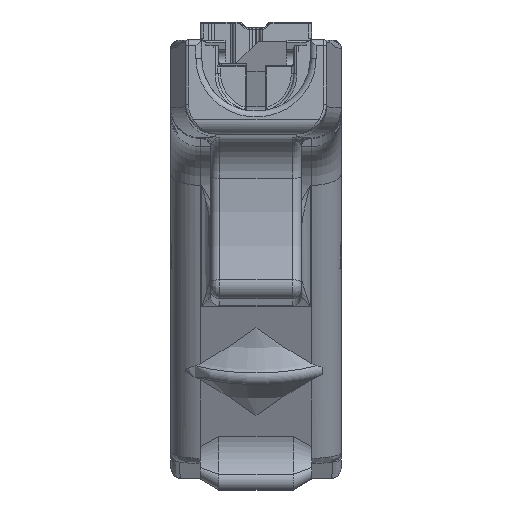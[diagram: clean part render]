
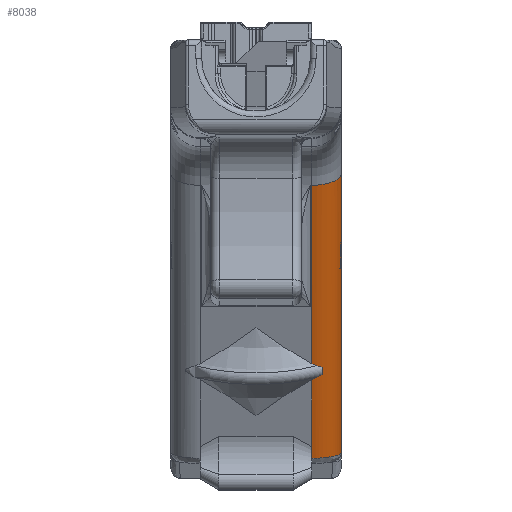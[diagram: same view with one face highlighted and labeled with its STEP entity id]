
A CAD part, top view. The second image highlights one B-rep face of the part: STEP entity #8038.
In plain terms, the highlighted cylindrical face has radius 5.08 mm (diameter 10.16 mm), a partial arc.
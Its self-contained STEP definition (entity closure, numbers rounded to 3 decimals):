
#89=(
BOUNDED_CURVE()
B_SPLINE_CURVE(3,(#33505,#33506,#33507,#33508,#33509,#33510,#33511,#33512,
#33513,#33514),.UNSPECIFIED.,.F.,.F.)
B_SPLINE_CURVE_WITH_KNOTS((4,2,2,2,4),(0.,0.393,0.785,
1.178,1.571),.UNSPECIFIED.)
CURVE()
GEOMETRIC_REPRESENTATION_ITEM()
RATIONAL_B_SPLINE_CURVE((1.,1.,1.,1.,1.,1.,1.,1.,1.,1.))
REPRESENTATION_ITEM('')
);
#125=ELLIPSE('',#8392,5.11,5.08);
#160=ELLIPSE('',#8741,46.774,5.08);
#799=LINE('',#29656,#1373);
#800=LINE('',#29658,#1374);
#846=LINE('',#32326,#1420);
#848=LINE('',#32330,#1422);
#899=LINE('',#33502,#1473);
#900=LINE('',#33504,#1474);
#1373=VECTOR('',#10200,1000.);
#1374=VECTOR('',#10201,1000.);
#1420=VECTOR('',#10403,1000.);
#1422=VECTOR('',#10407,1000.);
#1473=VECTOR('',#10572,1000.);
#1474=VECTOR('',#10573,1000.);
#1621=CYLINDRICAL_SURFACE('',#8740,5.08);
#1986=FACE_OUTER_BOUND('',#2454,.T.);
#2454=EDGE_LOOP('',(#7122,#7123,#7124,#7125,#7126,#7127,#7128,#7129,#7130,
#7131,#7132,#7133,#7134,#7135,#7136));
#2663=CIRCLE('',#8394,5.14);
#2814=CIRCLE('',#8739,5.08);
#3076=B_SPLINE_CURVE_WITH_KNOTS('',3,(#31899,#31900,#31901,#31902),
 .UNSPECIFIED.,.F.,.F.,(4,4),(3.929,4.031),
 .UNSPECIFIED.);
#3077=B_SPLINE_CURVE_WITH_KNOTS('',3,(#31905,#31906,#31907,#31908,#31909,
#31910),.UNSPECIFIED.,.F.,.F.,(4,2,4),(-0.097,-0.066,
-0.064),.UNSPECIFIED.);
#3078=B_SPLINE_CURVE_WITH_KNOTS('',3,(#31914,#31915,#31916,#31917,#31918,
#31919),.UNSPECIFIED.,.F.,.F.,(4,2,4),(-0.485,-0.459,
-0.454),.UNSPECIFIED.);
#3083=B_SPLINE_CURVE_WITH_KNOTS('',3,(#31967,#31968,#31969,#31970,#31971,
#31972),.UNSPECIFIED.,.F.,.F.,(4,2,4),(2.418,2.421,
2.517),.UNSPECIFIED.);
#3503=VERTEX_POINT('',#28126);
#3504=VERTEX_POINT('',#28128);
#3505=VERTEX_POINT('',#28132);
#3506=VERTEX_POINT('',#28134);
#3726=VERTEX_POINT('',#29654);
#3727=VERTEX_POINT('',#29657);
#3800=VERTEX_POINT('',#31878);
#3803=VERTEX_POINT('',#31892);
#3804=VERTEX_POINT('',#31904);
#3805=VERTEX_POINT('',#31911);
#3806=VERTEX_POINT('',#31913);
#3809=VERTEX_POINT('',#31949);
#3818=VERTEX_POINT('',#32324);
#3819=VERTEX_POINT('',#32329);
#3890=VERTEX_POINT('',#33503);
#4439=EDGE_CURVE('',#3503,#3504,#125,.T.);
#4442=EDGE_CURVE('',#3505,#3506,#2663,.T.);
#4789=EDGE_CURVE('',#3726,#3505,#799,.T.);
#4790=EDGE_CURVE('',#3504,#3727,#800,.T.);
#4893=EDGE_CURVE('',#3803,#3800,#3076,.T.);
#4894=EDGE_CURVE('',#3800,#3804,#3077,.T.);
#4896=EDGE_CURVE('',#3805,#3806,#3078,.T.);
#4902=EDGE_CURVE('',#3806,#3809,#3083,.T.);
#4922=EDGE_CURVE('',#3818,#3803,#846,.T.);
#4924=EDGE_CURVE('',#3809,#3819,#848,.T.);
#5033=EDGE_CURVE('',#3726,#3819,#2814,.T.);
#5034=EDGE_CURVE('',#3805,#3804,#899,.T.);
#5035=EDGE_CURVE('',#3890,#3818,#900,.T.);
#5036=EDGE_CURVE('',#3890,#3727,#89,.T.);
#5037=EDGE_CURVE('',#3506,#3503,#160,.T.);
#7122=ORIENTED_EDGE('',*,*,#4442,.F.);
#7123=ORIENTED_EDGE('',*,*,#4789,.F.);
#7124=ORIENTED_EDGE('',*,*,#5033,.T.);
#7125=ORIENTED_EDGE('',*,*,#4924,.F.);
#7126=ORIENTED_EDGE('',*,*,#4902,.F.);
#7127=ORIENTED_EDGE('',*,*,#4896,.F.);
#7128=ORIENTED_EDGE('',*,*,#5034,.T.);
#7129=ORIENTED_EDGE('',*,*,#4894,.F.);
#7130=ORIENTED_EDGE('',*,*,#4893,.F.);
#7131=ORIENTED_EDGE('',*,*,#4922,.F.);
#7132=ORIENTED_EDGE('',*,*,#5035,.F.);
#7133=ORIENTED_EDGE('',*,*,#5036,.T.);
#7134=ORIENTED_EDGE('',*,*,#4790,.F.);
#7135=ORIENTED_EDGE('',*,*,#4439,.F.);
#7136=ORIENTED_EDGE('',*,*,#5037,.F.);
#8038=ADVANCED_FACE('',(#1986),#1621,.T.);
#8392=AXIS2_PLACEMENT_3D('',#28129,#9583,#9584);
#8394=AXIS2_PLACEMENT_3D('',#28135,#9589,#9590);
#8739=AXIS2_PLACEMENT_3D('',#33500,#10568,#10569);
#8740=AXIS2_PLACEMENT_3D('',#33501,#10570,#10571);
#8741=AXIS2_PLACEMENT_3D('',#33515,#10574,#10575);
#9583=DIRECTION('center_axis',(0.,0.952,0.305));
#9584=DIRECTION('ref_axis',(0.,-0.305,0.952));
#9589=DIRECTION('center_axis',(0.,-0.952,
-0.305));
#9590=DIRECTION('ref_axis',(0.995,-0.03,0.093));
#10200=DIRECTION('',(0.,-0.914,-0.407));
#10201=DIRECTION('',(0.,-0.914,-0.407));
#10403=DIRECTION('',(0.,0.914,0.407));
#10407=DIRECTION('',(0.,0.914,0.407));
#10568=DIRECTION('center_axis',(0.,-0.914,-0.407));
#10569=DIRECTION('ref_axis',(0.,0.407,-0.914));
#10570=DIRECTION('center_axis',(0.,0.914,0.407));
#10571=DIRECTION('ref_axis',(0.,-0.407,0.914));
#10572=DIRECTION('',(0.,-0.914,-0.407));
#10573=DIRECTION('',(0.,0.914,0.407));
#10574=DIRECTION('center_axis',(0.,0.305,
-0.952));
#10575=DIRECTION('ref_axis',(0.,0.952,0.305));
#28126=CARTESIAN_POINT('',(14.424,-38.99,-96.538));
#28128=CARTESIAN_POINT('',(14.605,-38.578,-97.825));
#28129=CARTESIAN_POINT('Origin',(9.525,-38.578,-97.825));
#28132=CARTESIAN_POINT('',(14.605,-31.459,-94.656));
#28134=CARTESIAN_POINT('',(14.58,-31.613,-94.175));
#28135=CARTESIAN_POINT('Origin',(9.465,-31.459,-94.656));
#29654=CARTESIAN_POINT('',(14.605,-22.676,-90.746));
#29656=CARTESIAN_POINT('',(14.605,-70.324,-111.956));
#29657=CARTESIAN_POINT('',(14.605,-70.353,-111.969));
#29658=CARTESIAN_POINT('',(14.605,-70.324,-111.956));
#31878=CARTESIAN_POINT('',(10.428,-57.542,-100.794));
#31892=CARTESIAN_POINT('',(9.525,-57.963,-100.893));
#31899=CARTESIAN_POINT('Ctrl Pts',(9.525,-57.963,-100.893));
#31900=CARTESIAN_POINT('Ctrl Pts',(9.817,-57.812,-100.826));
#31901=CARTESIAN_POINT('Ctrl Pts',(10.12,-57.673,-100.792));
#31902=CARTESIAN_POINT('Ctrl Pts',(10.428,-57.542,-100.794));
#31904=CARTESIAN_POINT('',(11.329,-57.063,-100.855));
#31905=CARTESIAN_POINT('Ctrl Pts',(10.428,-57.542,-100.794));
#31906=CARTESIAN_POINT('Ctrl Pts',(10.749,-57.405,-100.797));
#31907=CARTESIAN_POINT('Ctrl Pts',(11.038,-57.249,-100.82));
#31908=CARTESIAN_POINT('Ctrl Pts',(11.298,-57.082,-100.851));
#31909=CARTESIAN_POINT('Ctrl Pts',(11.314,-57.073,-100.853));
#31910=CARTESIAN_POINT('Ctrl Pts',(11.329,-57.063,-100.855));
#31911=CARTESIAN_POINT('',(11.329,-55.855,-100.317));
#31913=CARTESIAN_POINT('',(10.428,-55.58,-99.921));
#31914=CARTESIAN_POINT('Ctrl Pts',(11.329,-55.855,-100.317));
#31915=CARTESIAN_POINT('Ctrl Pts',(11.127,-55.786,-100.202));
#31916=CARTESIAN_POINT('Ctrl Pts',(10.879,-55.709,-100.081));
#31917=CARTESIAN_POINT('Ctrl Pts',(10.539,-55.611,-99.958));
#31918=CARTESIAN_POINT('Ctrl Pts',(10.484,-55.595,-99.939));
#31919=CARTESIAN_POINT('Ctrl Pts',(10.428,-55.58,-99.921));
#31949=CARTESIAN_POINT('',(9.525,-55.224,-99.674));
#31967=CARTESIAN_POINT('Ctrl Pts',(10.428,-55.58,-99.921));
#31968=CARTESIAN_POINT('Ctrl Pts',(10.422,-55.578,-99.919));
#31969=CARTESIAN_POINT('Ctrl Pts',(10.415,-55.576,-99.917));
#31970=CARTESIAN_POINT('Ctrl Pts',(10.107,-55.489,-99.818));
#31971=CARTESIAN_POINT('Ctrl Pts',(9.811,-55.372,-99.74));
#31972=CARTESIAN_POINT('Ctrl Pts',(9.525,-55.224,-99.674));
#32324=CARTESIAN_POINT('',(9.525,-69.405,-105.986));
#32326=CARTESIAN_POINT('',(9.525,-24.741,-86.105));
#32329=CARTESIAN_POINT('',(9.525,-24.741,-86.105));
#32330=CARTESIAN_POINT('',(9.525,-24.741,-86.105));
#33500=CARTESIAN_POINT('Origin',(9.525,-22.676,-90.746));
#33501=CARTESIAN_POINT('Origin',(9.525,17.678,-72.784));
#33502=CARTESIAN_POINT('',(11.329,15.747,-68.445));
#33503=CARTESIAN_POINT('',(9.525,-71.375,-106.863));
#33504=CARTESIAN_POINT('',(9.525,-24.741,-86.105));
#33505=CARTESIAN_POINT('Ctrl Pts',(9.525,-71.375,-106.863));
#33506=CARTESIAN_POINT('Ctrl Pts',(10.19,-71.375,-106.863));
#33507=CARTESIAN_POINT('Ctrl Pts',(10.855,-71.348,-106.996));
#33508=CARTESIAN_POINT('Ctrl Pts',(12.083,-71.246,-107.508));
#33509=CARTESIAN_POINT('Ctrl Pts',(12.647,-71.17,-107.886));
#33510=CARTESIAN_POINT('Ctrl Pts',(13.587,-70.981,-108.831));
#33511=CARTESIAN_POINT('Ctrl Pts',(13.964,-70.868,-109.398));
#33512=CARTESIAN_POINT('Ctrl Pts',(14.473,-70.621,-110.633));
#33513=CARTESIAN_POINT('Ctrl Pts',(14.605,-70.487,-111.301));
#33514=CARTESIAN_POINT('Ctrl Pts',(14.605,-70.353,-111.969));
#33515=CARTESIAN_POINT('Origin',(9.525,-27.214,-92.766));
